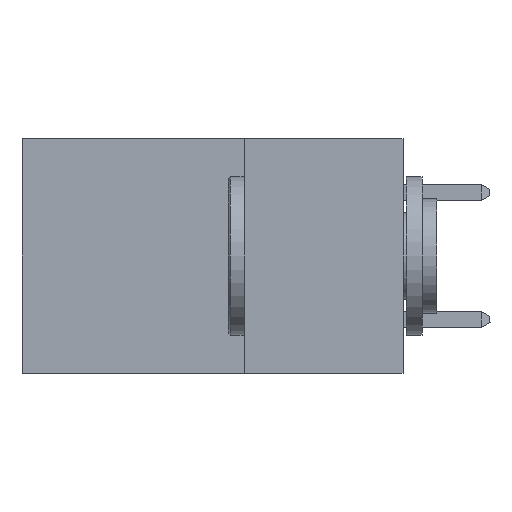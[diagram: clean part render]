
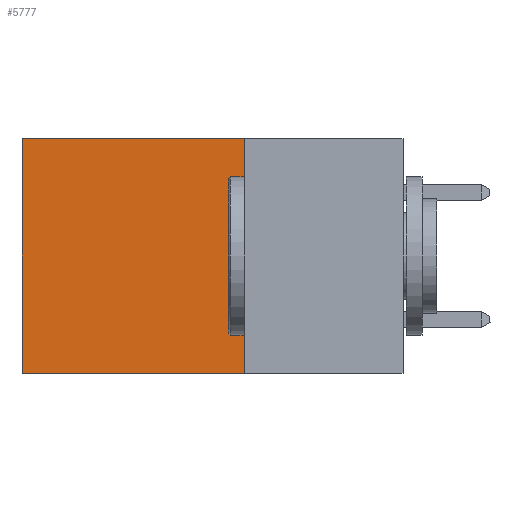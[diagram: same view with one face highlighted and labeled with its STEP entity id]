
A CAD part, left-side view. The second image highlights one B-rep face of the part: STEP entity #5777.
In plain terms, the highlighted planar face has unit normal (-1, 0, 0).
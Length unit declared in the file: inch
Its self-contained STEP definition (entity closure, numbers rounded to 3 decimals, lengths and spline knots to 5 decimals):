
#358 = FACE_OUTER_BOUND ( 'NONE', #8614, .T. ) ;
#765 = ORIENTED_EDGE ( 'NONE', *, *, #3466, .T. ) ;
#892 = CARTESIAN_POINT ( 'NONE',  ( 0.2875, 0.25, -0.37 ) ) ;
#1697 = CARTESIAN_POINT ( 'NONE',  ( 0.2875, 0.6, 0. ) ) ;
#2580 = VECTOR ( 'NONE', #4446, 39.37008 ) ;
#2927 = VECTOR ( 'NONE', #5506, 39.37008 ) ;
#3123 = DIRECTION ( 'NONE',  ( 1., 0., 0. ) ) ;
#3126 = EDGE_CURVE ( 'NONE', #9225, #8459, #12210, .T. ) ;
#3431 = EDGE_CURVE ( 'NONE', #9225, #4398, #6960, .T. ) ;
#3466 = EDGE_CURVE ( 'NONE', #8459, #8339, #5879, .T. ) ;
#3490 = CARTESIAN_POINT ( 'NONE',  ( 0.2875, 0.25, 0. ) ) ;
#4198 = CARTESIAN_POINT ( 'NONE',  ( 0.2875, 0.6, -0.37 ) ) ;
#4313 = VECTOR ( 'NONE', #6142, 39.37008 ) ;
#4398 = VERTEX_POINT ( 'NONE', #892 ) ;
#4446 = DIRECTION ( 'NONE',  ( 0., 0., -1. ) ) ;
#5125 = CARTESIAN_POINT ( 'NONE',  ( 0.2875, 0.25, 0. ) ) ;
#5202 = EDGE_CURVE ( 'NONE', #4398, #8339, #8131, .T. ) ;
#5506 = DIRECTION ( 'NONE',  ( 0., 1., 0. ) ) ;
#5777 = ADVANCED_FACE ( 'NONE', ( #358 ), #11982, .F. ) ;
#5879 = LINE ( 'NONE', #11322, #2580 ) ;
#5902 = CARTESIAN_POINT ( 'NONE',  ( 0.2875, 0.25, -0.37 ) ) ;
#6046 = CARTESIAN_POINT ( 'NONE',  ( 0.2875, 0.25, 0. ) ) ;
#6142 = DIRECTION ( 'NONE',  ( 0., 0., -1. ) ) ;
#6183 = CARTESIAN_POINT ( 'NONE',  ( 0.2875, 0.25, 0. ) ) ;
#6960 = LINE ( 'NONE', #5125, #4313 ) ;
#8131 = LINE ( 'NONE', #5902, #9827 ) ;
#8281 = AXIS2_PLACEMENT_3D ( 'NONE', #6046, #3123, #8969 ) ;
#8339 = VERTEX_POINT ( 'NONE', #4198 ) ;
#8459 = VERTEX_POINT ( 'NONE', #1697 ) ;
#8614 = EDGE_LOOP ( 'NONE', ( #765, #11267, #11206, #12776 ) ) ;
#8863 = DIRECTION ( 'NONE',  ( 0., 1., 0. ) ) ;
#8969 = DIRECTION ( 'NONE',  ( 0., 0., -1. ) ) ;
#9225 = VERTEX_POINT ( 'NONE', #6183 ) ;
#9827 = VECTOR ( 'NONE', #8863, 39.37008 ) ;
#11206 = ORIENTED_EDGE ( 'NONE', *, *, #3431, .F. ) ;
#11267 = ORIENTED_EDGE ( 'NONE', *, *, #5202, .F. ) ;
#11322 = CARTESIAN_POINT ( 'NONE',  ( 0.2875, 0.6, 0. ) ) ;
#11982 = PLANE ( 'NONE',  #8281 ) ;
#12210 = LINE ( 'NONE', #3490, #2927 ) ;
#12776 = ORIENTED_EDGE ( 'NONE', *, *, #3126, .T. ) ;
